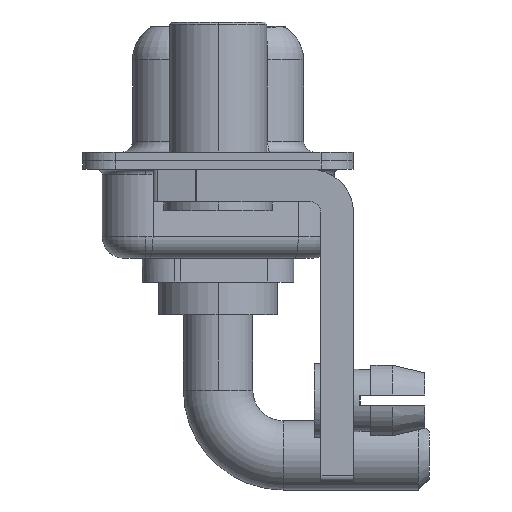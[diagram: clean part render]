
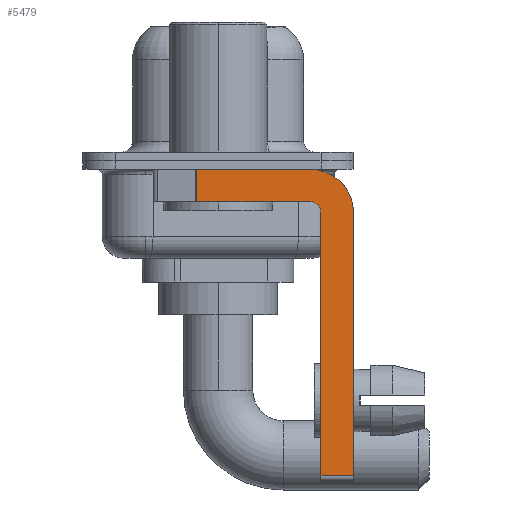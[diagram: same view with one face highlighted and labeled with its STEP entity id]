
A CAD part, left-side view. The second image highlights one B-rep face of the part: STEP entity #5479.
In plain terms, the highlighted planar face has unit normal (-1, 0, 0).
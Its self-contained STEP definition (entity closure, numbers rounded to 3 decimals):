
#117 = DIRECTION ( 'NONE',  ( -1., 0., 0. ) ) ;
#184 = VERTEX_POINT ( 'NONE', #13314 ) ;
#652 = DIRECTION ( 'NONE',  ( 0., 0., 1. ) ) ;
#1253 = CARTESIAN_POINT ( 'NONE',  ( -2.9, -4.25, -1.9 ) ) ;
#1422 = DIRECTION ( 'NONE',  ( 0., 0., -1. ) ) ;
#1423 = CARTESIAN_POINT ( 'NONE',  ( -2.9, -4.75, -14.55 ) ) ;
#1427 = AXIS2_PLACEMENT_3D ( 'NONE', #1582, #15085, #1422 ) ;
#1494 = CIRCLE ( 'NONE', #13033, 0.5 ) ;
#1582 = CARTESIAN_POINT ( 'NONE',  ( -2.9, -4.25, -2.4 ) ) ;
#2026 = DIRECTION ( 'NONE',  ( 0., -1., 0. ) ) ;
#2085 = LINE ( 'NONE', #2155, #2539 ) ;
#2155 = CARTESIAN_POINT ( 'NONE',  ( -2.9, 0.978, -1.9 ) ) ;
#2539 = VECTOR ( 'NONE', #7082, 1000. ) ;
#2796 = ORIENTED_EDGE ( 'NONE', *, *, #4119, .F. ) ;
#3205 = CARTESIAN_POINT ( 'NONE',  ( -2.9, -4.75, -14.8 ) ) ;
#3255 = VECTOR ( 'NONE', #4109, 1000. ) ;
#3434 = CARTESIAN_POINT ( 'NONE',  ( -2.9, -6.25, -2.4 ) ) ;
#3717 = ORIENTED_EDGE ( 'NONE', *, *, #15201, .F. ) ;
#4018 = VERTEX_POINT ( 'NONE', #14941 ) ;
#4109 = DIRECTION ( 'NONE',  ( 0., -1., 0. ) ) ;
#4119 = EDGE_CURVE ( 'NONE', #11692, #8266, #6501, .T. ) ;
#4568 = ORIENTED_EDGE ( 'NONE', *, *, #10770, .F. ) ;
#4826 = VERTEX_POINT ( 'NONE', #13210 ) ;
#5031 = DIRECTION ( 'NONE',  ( 0., 0., 1. ) ) ;
#5357 = DIRECTION ( 'NONE',  ( 0., 0., -1. ) ) ;
#5479 = ADVANCED_FACE ( 'NONE', ( #6558 ), #11705, .F. ) ;
#5551 = CARTESIAN_POINT ( 'NONE',  ( -2.9, -6.25, -14.55 ) ) ;
#5649 = AXIS2_PLACEMENT_3D ( 'NONE', #11468, #6638, #5357 ) ;
#5894 = ORIENTED_EDGE ( 'NONE', *, *, #14360, .F. ) ;
#6501 = LINE ( 'NONE', #10442, #14433 ) ;
#6558 = FACE_OUTER_BOUND ( 'NONE', #7778, .T. ) ;
#6586 = VECTOR ( 'NONE', #9958, 1000. ) ;
#6638 = DIRECTION ( 'NONE',  ( 1., 0., 0. ) ) ;
#6666 = EDGE_CURVE ( 'NONE', #12273, #8266, #10806, .T. ) ;
#7082 = DIRECTION ( 'NONE',  ( 0., 0., -1. ) ) ;
#7778 = EDGE_LOOP ( 'NONE', ( #11655, #13441, #3717, #4568, #9427, #13680, #2796, #5894 ) ) ;
#8266 = VERTEX_POINT ( 'NONE', #5551 ) ;
#8353 = CIRCLE ( 'NONE', #1427, 2. ) ;
#8779 = VERTEX_POINT ( 'NONE', #14688 ) ;
#9031 = VECTOR ( 'NONE', #2026, 1000. ) ;
#9427 = ORIENTED_EDGE ( 'NONE', *, *, #11577, .F. ) ;
#9914 = EDGE_CURVE ( 'NONE', #10938, #8779, #13847, .T. ) ;
#9953 = CARTESIAN_POINT ( 'NONE',  ( -2.9, -4.25, -2.4 ) ) ;
#9958 = DIRECTION ( 'NONE',  ( 0., 1., 0. ) ) ;
#10261 = VECTOR ( 'NONE', #652, 1000. ) ;
#10405 = CARTESIAN_POINT ( 'NONE',  ( -2.9, 0.978, -0.4 ) ) ;
#10442 = CARTESIAN_POINT ( 'NONE',  ( -2.9, -6.25, -2.4 ) ) ;
#10706 = LINE ( 'NONE', #3205, #10261 ) ;
#10770 = EDGE_CURVE ( 'NONE', #184, #4826, #1494, .T. ) ;
#10806 = LINE ( 'NONE', #10880, #9031 ) ;
#10880 = CARTESIAN_POINT ( 'NONE',  ( -2.9, -4.25, -14.55 ) ) ;
#10938 = VERTEX_POINT ( 'NONE', #10405 ) ;
#11468 = CARTESIAN_POINT ( 'NONE',  ( -2.9, -4.25, -2.4 ) ) ;
#11555 = EDGE_CURVE ( 'NONE', #10938, #4018, #2085, .T. ) ;
#11577 = EDGE_CURVE ( 'NONE', #12273, #184, #10706, .T. ) ;
#11655 = ORIENTED_EDGE ( 'NONE', *, *, #9914, .F. ) ;
#11692 = VERTEX_POINT ( 'NONE', #3434 ) ;
#11705 = PLANE ( 'NONE',  #5649 ) ;
#12273 = VERTEX_POINT ( 'NONE', #1423 ) ;
#12633 = CARTESIAN_POINT ( 'NONE',  ( -2.9, 3., -0.4 ) ) ;
#12686 = DIRECTION ( 'NONE',  ( 0., 0., -1. ) ) ;
#13033 = AXIS2_PLACEMENT_3D ( 'NONE', #9953, #117, #5031 ) ;
#13210 = CARTESIAN_POINT ( 'NONE',  ( -2.9, -4.25, -1.9 ) ) ;
#13314 = CARTESIAN_POINT ( 'NONE',  ( -2.9, -4.75, -2.4 ) ) ;
#13441 = ORIENTED_EDGE ( 'NONE', *, *, #11555, .T. ) ;
#13640 = LINE ( 'NONE', #1253, #6586 ) ;
#13680 = ORIENTED_EDGE ( 'NONE', *, *, #6666, .T. ) ;
#13847 = LINE ( 'NONE', #12633, #3255 ) ;
#14360 = EDGE_CURVE ( 'NONE', #8779, #11692, #8353, .T. ) ;
#14433 = VECTOR ( 'NONE', #12686, 1000. ) ;
#14688 = CARTESIAN_POINT ( 'NONE',  ( -2.9, -4.25, -0.4 ) ) ;
#14941 = CARTESIAN_POINT ( 'NONE',  ( -2.9, 0.978, -1.9 ) ) ;
#15085 = DIRECTION ( 'NONE',  ( 1., 0., 0. ) ) ;
#15201 = EDGE_CURVE ( 'NONE', #4826, #4018, #13640, .T. ) ;
